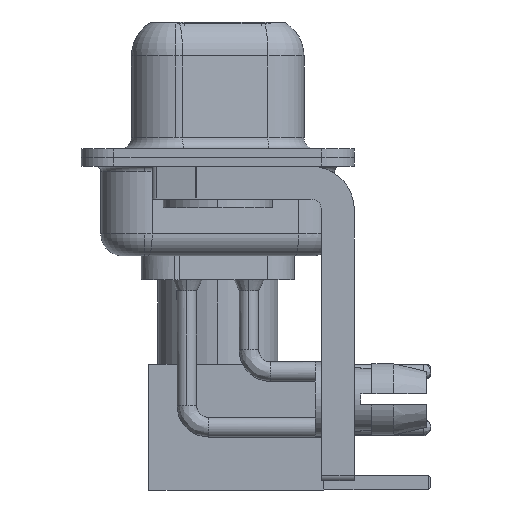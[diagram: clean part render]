
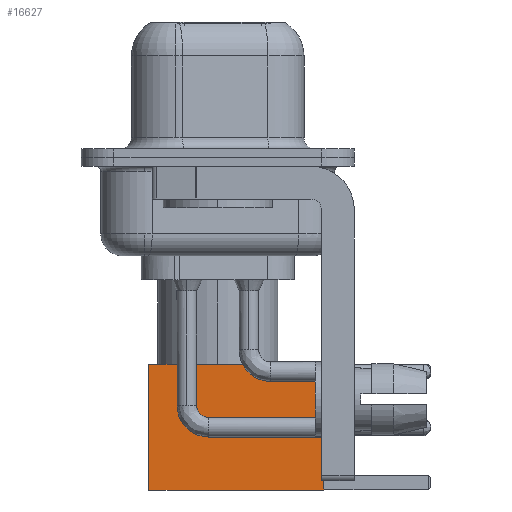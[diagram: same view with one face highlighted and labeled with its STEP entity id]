
A CAD part, left-side view. The second image highlights one B-rep face of the part: STEP entity #16627.
In plain terms, the highlighted face is planar.
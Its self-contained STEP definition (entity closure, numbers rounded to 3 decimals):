
#31 = EDGE_CURVE ( 'NONE', #14327, #12910, #8262, .T. ) ;
#581 = PLANE ( 'NONE',  #2767 ) ;
#2680 = CARTESIAN_POINT ( 'NONE',  ( 0., 2.875, 8. ) ) ;
#2767 = AXIS2_PLACEMENT_3D ( 'NONE', #4340, #14290, #19373 ) ;
#3551 = DIRECTION ( 'NONE',  ( 0., 0., -1. ) ) ;
#3612 = CARTESIAN_POINT ( 'NONE',  ( -2.875, 2.875, 0. ) ) ;
#3971 = ORIENTED_EDGE ( 'NONE', *, *, #31, .F. ) ;
#4340 = CARTESIAN_POINT ( 'NONE',  ( 2.875, 2.875, 0. ) ) ;
#4935 = ORIENTED_EDGE ( 'NONE', *, *, #20210, .T. ) ;
#5971 = ORIENTED_EDGE ( 'NONE', *, *, #18319, .T. ) ;
#7027 = VECTOR ( 'NONE', #18530, 1000. ) ;
#8262 = LINE ( 'NONE', #3612, #7027 ) ;
#8544 = VECTOR ( 'NONE', #9211, 1000. ) ;
#8621 = CARTESIAN_POINT ( 'NONE',  ( -2.875, 2.875, 0. ) ) ;
#9211 = DIRECTION ( 'NONE',  ( -1., 0., 0. ) ) ;
#9451 = CARTESIAN_POINT ( 'NONE',  ( 0., 2.875, 0. ) ) ;
#10411 = EDGE_LOOP ( 'NONE', ( #5971, #4935, #3971, #20202 ) ) ;
#11090 = LINE ( 'NONE', #2680, #8544 ) ;
#11749 = CARTESIAN_POINT ( 'NONE',  ( -2.875, 2.875, 8. ) ) ;
#12673 = DIRECTION ( 'NONE',  ( -1., 0., 0. ) ) ;
#12753 = FACE_OUTER_BOUND ( 'NONE', #10411, .T. ) ;
#12910 = VERTEX_POINT ( 'NONE', #8621 ) ;
#13137 = VECTOR ( 'NONE', #12673, 1000. ) ;
#14290 = DIRECTION ( 'NONE',  ( 0., 1., 0. ) ) ;
#14327 = VERTEX_POINT ( 'NONE', #11749 ) ;
#14779 = VERTEX_POINT ( 'NONE', #19966 ) ;
#15047 = VERTEX_POINT ( 'NONE', #18790 ) ;
#16627 = ADVANCED_FACE ( 'NONE', ( #12753 ), #581, .T. ) ;
#18059 = LINE ( 'NONE', #9451, #13137 ) ;
#18319 = EDGE_CURVE ( 'NONE', #15047, #14779, #20660, .T. ) ;
#18530 = DIRECTION ( 'NONE',  ( 0., 0., -1. ) ) ;
#18790 = CARTESIAN_POINT ( 'NONE',  ( 2.875, 2.875, 8. ) ) ;
#19373 = DIRECTION ( 'NONE',  ( 0., 0., 1. ) ) ;
#19761 = VECTOR ( 'NONE', #3551, 1000. ) ;
#19966 = CARTESIAN_POINT ( 'NONE',  ( 2.875, 2.875, 0. ) ) ;
#20202 = ORIENTED_EDGE ( 'NONE', *, *, #20729, .F. ) ;
#20210 = EDGE_CURVE ( 'NONE', #14779, #12910, #18059, .T. ) ;
#20338 = CARTESIAN_POINT ( 'NONE',  ( 2.875, 2.875, 0. ) ) ;
#20660 = LINE ( 'NONE', #20338, #19761 ) ;
#20729 = EDGE_CURVE ( 'NONE', #15047, #14327, #11090, .T. ) ;
